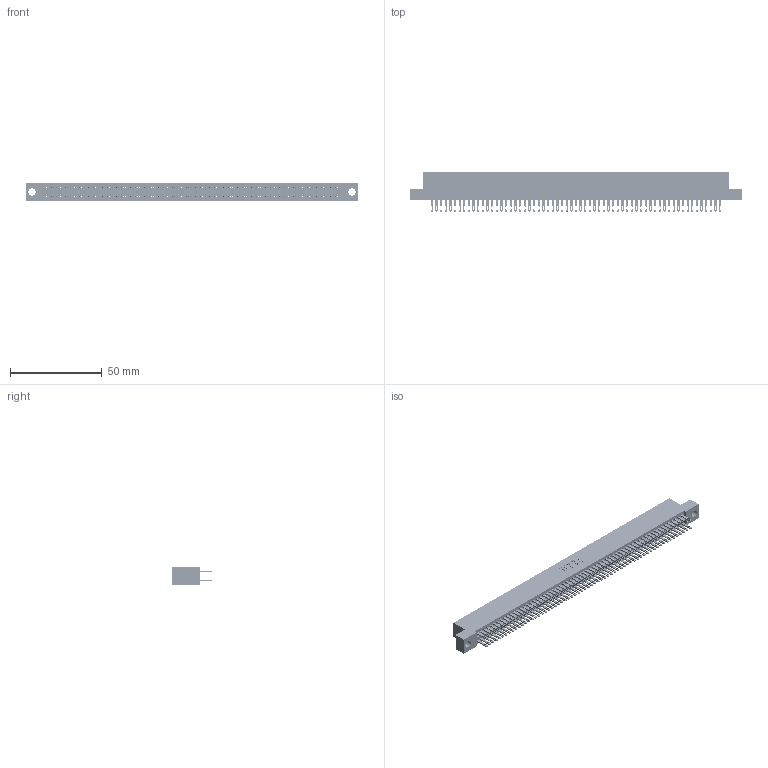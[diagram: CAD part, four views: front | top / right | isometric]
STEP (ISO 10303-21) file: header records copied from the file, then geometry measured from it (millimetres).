
FILE_DESCRIPTION (( 'STEP AP203' ), '1' );
FILE_NAME ('345-126-500-204.STEP', '2021-05-25T18:46:33', ( '' ), ( '' ), 'SwSTEP 2.0', 'SolidWorks 2020', '' );
FILE_SCHEMA (( 'CONFIG_CONTROL_DESIGN' ));
Length unit declared in the file: inch
Products named in the file (3): 345-126-500-204; 345-292-001_345-293-100; 345 Part_Flush Mounting Lugs - 0.156 Dia-TI
Assembly tree (127 placements, depth 2):
  345-126-500-204
    345 Part_Flush Mounting Lugs - 0.156 Dia-TI
    345-292-001_345-293-100  x126
Bounding box: 181.23 x 21.51 x 9.4 mm (x, y, z)
Volume: 18078.8 mm3; surface area: 28266.9 mm2
Topology: 127 solids, 127 shells, 5936 faces, 18143 edges, 12094 vertices
Faces by surface type: plane 3496, cylinder 2440
Entity records: 46953 total; most frequent: CARTESIAN_POINT 7854, ORIENTED_EDGE 7786, DIRECTION 6901, EDGE_CURVE 3893, VECTOR 3505, LINE 3505, VERTEX_POINT 2594, AXIS2_PLACEMENT_3D 1698
